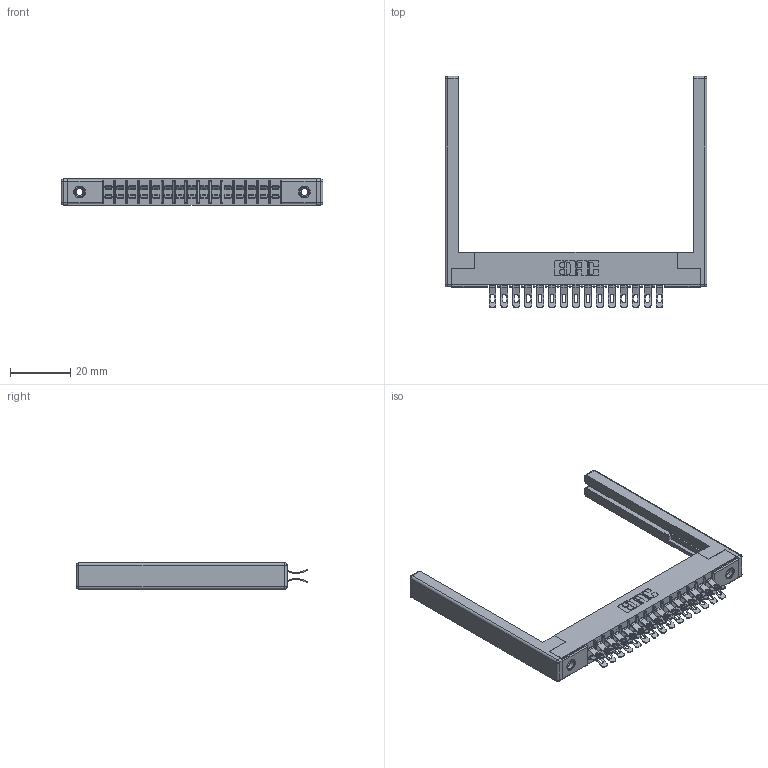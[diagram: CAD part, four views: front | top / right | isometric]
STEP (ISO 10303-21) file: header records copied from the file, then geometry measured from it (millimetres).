
FILE_DESCRIPTION (( 'STEP AP203' ), '1' );
FILE_NAME ('355-030-555-568.STEP', '2019-09-11T07:23:21', ( '' ), ( '' ), 'SwSTEP 2.0', 'SolidWorks 2016', '' );
FILE_SCHEMA (( 'CONFIG_CONTROL_DESIGN' ));
Length unit declared in the file: inch
Products named in the file (5): 355-030-555-568; 305-290-001_555; 345-250-001_345-250-001-102; 307-220-068; 305 Part_.156 Dia
Assembly tree (35 placements, depth 2):
  355-030-555-568
    305 Part_.156 Dia
    305-290-001_555  x30
    345-250-001_345-250-001-102  x2
    307-220-068  x2
Bounding box: 86.87 x 76.71 x 8.71 mm (x, y, z)
Volume: 9907.5 mm3; surface area: 14680.2 mm2
Topology: 35 solids, 35 shells, 2250 faces, 6631 edges, 4318 vertices
Faces by surface type: plane 1116, cylinder 1050, sphere 68, cone 12, torus 4
Entity records: 22911 total; most frequent: CARTESIAN_POINT 3782, ORIENTED_EDGE 3732, DIRECTION 3694, EDGE_CURVE 1866, LINE 1450, VECTOR 1450, VERTEX_POINT 1194, AXIS2_PLACEMENT_3D 1122
